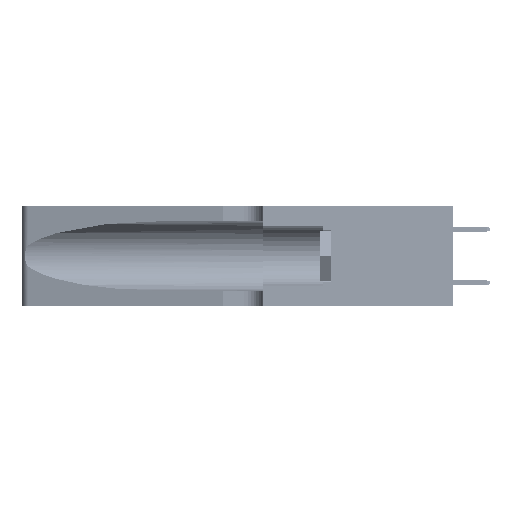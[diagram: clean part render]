
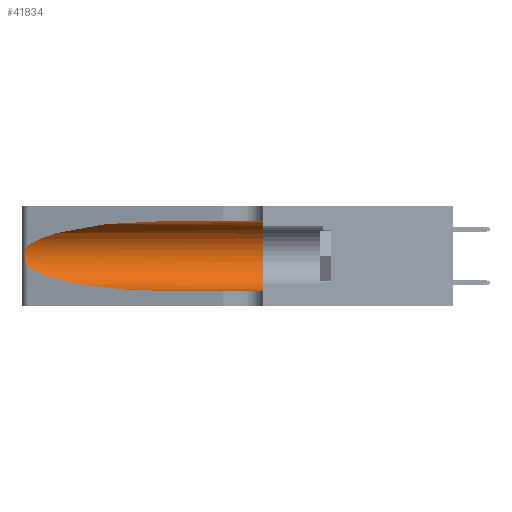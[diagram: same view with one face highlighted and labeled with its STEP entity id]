
A CAD part, left-side view. The second image highlights one B-rep face of the part: STEP entity #41834.
In plain terms, the highlighted cylindrical face has radius 3.308 mm (diameter 6.617 mm), a partial arc.
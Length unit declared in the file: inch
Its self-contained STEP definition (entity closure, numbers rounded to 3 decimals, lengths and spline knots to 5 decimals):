
#652 = FACE_OUTER_BOUND ( 'NONE', #35415, .T. ) ;
#1297 = ORIENTED_EDGE ( 'NONE', *, *, #24141, .F. ) ;
#1876 = EDGE_CURVE ( 'NONE', #30815, #19886, #15524, .T. ) ;
#3003 = CARTESIAN_POINT ( 'NONE',  ( 0.1305, 0.35, 0.31525 ) ) ;
#4019 = CARTESIAN_POINT ( 'NONE',  ( 0.1305, 0.72297, 0.31525 ) ) ;
#4290 = DIRECTION ( 'NONE',  ( 0., 0., -1. ) ) ;
#4959 = AXIS2_PLACEMENT_3D ( 'NONE', #5376, #8718, #4290 ) ;
#5376 = CARTESIAN_POINT ( 'NONE',  ( 0.1305, 1.61858, 0.185 ) ) ;
#7870 = CARTESIAN_POINT ( 'NONE',  ( 0.25854, 1.2359, 0.20912 ) ) ;
#8489 = VERTEX_POINT ( 'NONE', #17965 ) ;
#8718 = DIRECTION ( 'NONE',  ( 0., -1., 0. ) ) ;
#8997 = CYLINDRICAL_SURFACE ( 'NONE', #4959, 0.13025 ) ;
#9304 = CARTESIAN_POINT ( 'NONE',  ( 0.1305, 1.61858, 0.31525 ) ) ;
#9353 = B_SPLINE_CURVE_WITH_KNOTS ( 'NONE', 3,
 ( #24825, #20412, #28761, #49538, #7870, #41749, #29020, #24554, #20707, #45372, #40950, #37334, #45639, #45912 ),
 .UNSPECIFIED., .F., .F.,
 ( 4, 2, 2, 2, 2, 2, 4 ),
 ( 0., 0.00027, 0.00053, 0.00107, 0.0016, 0.00187, 0.00214 ),
 .UNSPECIFIED. ) ;
#12402 = DIRECTION ( 'NONE',  ( 0., 0., 1. ) ) ;
#15524 =( BOUNDED_CURVE ( )  B_SPLINE_CURVE ( 3, ( #38106, #30896, #17821, #39204 ),
 .UNSPECIFIED., .F., .F. ) 
 B_SPLINE_CURVE_WITH_KNOTS ( ( 4, 4 ),
 ( 3.44316, 4.71239 ),
 .UNSPECIFIED. ) 
 CURVE ( )  GEOMETRIC_REPRESENTATION_ITEM ( )  RATIONAL_B_SPLINE_CURVE ( ( 1., 0.87, 0.87, 1. ) ) 
 REPRESENTATION_ITEM ( '' )  );
#17821 = CARTESIAN_POINT ( 'NONE',  ( 0.18966, 0.96281, 0.05475 ) ) ;
#17965 = CARTESIAN_POINT ( 'NONE',  ( 0.1305, 0.35, 0.05475 ) ) ;
#19604 = CARTESIAN_POINT ( 'NONE',  ( 0.1305, 0.72297, 0.31525 ) ) ;
#19886 = VERTEX_POINT ( 'NONE', #39700 ) ;
#20171 = EDGE_CURVE ( 'NONE', #38620, #42905, #29901, .T. ) ;
#20412 = CARTESIAN_POINT ( 'NONE',  ( 0.25555, 1.22994, 0.2215 ) ) ;
#20615 = ORIENTED_EDGE ( 'NONE', *, *, #26371, .T. ) ;
#20707 = CARTESIAN_POINT ( 'NONE',  ( 0.26017, 1.23833, 0.17102 ) ) ;
#20763 = CARTESIAN_POINT ( 'NONE',  ( 0.25487, 1.22718, 0.22369 ) ) ;
#21088 = ORIENTED_EDGE ( 'NONE', *, *, #1876, .T. ) ;
#21697 = CARTESIAN_POINT ( 'NONE',  ( 0.1305, 1.61858, 0.05475 ) ) ;
#21811 = DIRECTION ( 'NONE',  ( 0., 1., 0. ) ) ;
#24032 = CARTESIAN_POINT ( 'NONE',  ( 0.25487, 1.22718, 0.22369 ) ) ;
#24141 = EDGE_CURVE ( 'NONE', #42905, #8489, #38104, .T. ) ;
#24554 = CARTESIAN_POINT ( 'NONE',  ( 0.26075, 1.23896, 0.178 ) ) ;
#24825 = CARTESIAN_POINT ( 'NONE',  ( 0.25487, 1.22718, 0.22369 ) ) ;
#26371 = EDGE_CURVE ( 'NONE', #19886, #8489, #42766, .T. ) ;
#28761 = CARTESIAN_POINT ( 'NONE',  ( 0.25639, 1.23184, 0.21858 ) ) ;
#29020 = CARTESIAN_POINT ( 'NONE',  ( 0.26075, 1.23896, 0.19203 ) ) ;
#29901 = LINE ( 'NONE', #9304, #48557 ) ;
#30815 = VERTEX_POINT ( 'NONE', #36262 ) ;
#30896 = CARTESIAN_POINT ( 'NONE',  ( 0.2373, 1.15595, 0.08982 ) ) ;
#31035 = AXIS2_PLACEMENT_3D ( 'NONE', #46506, #21811, #12402 ) ;
#32673 = CARTESIAN_POINT ( 'NONE',  ( 0.2373, 1.15595, 0.28018 ) ) ;
#33665 = ORIENTED_EDGE ( 'NONE', *, *, #45540, .T. ) ;
#35415 = EDGE_LOOP ( 'NONE', ( #37313, #33665, #21088, #20615, #1297, #46848 ) ) ;
#36262 = CARTESIAN_POINT ( 'NONE',  ( 0.25487, 1.22718, 0.14631 ) ) ;
#37313 = ORIENTED_EDGE ( 'NONE', *, *, #49734, .T. ) ;
#37334 = CARTESIAN_POINT ( 'NONE',  ( 0.25639, 1.23186, 0.15144 ) ) ;
#38104 = CIRCLE ( 'NONE', #31035, 0.13025 ) ;
#38106 = CARTESIAN_POINT ( 'NONE',  ( 0.25487, 1.22718, 0.14631 ) ) ;
#38620 = VERTEX_POINT ( 'NONE', #4019 ) ;
#39204 = CARTESIAN_POINT ( 'NONE',  ( 0.1305, 0.72297, 0.05475 ) ) ;
#39700 = CARTESIAN_POINT ( 'NONE',  ( 0.1305, 0.72297, 0.05475 ) ) ;
#40950 = CARTESIAN_POINT ( 'NONE',  ( 0.25789, 1.23486, 0.15765 ) ) ;
#41499 = CARTESIAN_POINT ( 'NONE',  ( 0.18966, 0.96281, 0.31525 ) ) ;
#41749 = CARTESIAN_POINT ( 'NONE',  ( 0.26018, 1.23835, 0.19895 ) ) ;
#41834 = ADVANCED_FACE ( 'NONE', ( #652 ), #8997, .F. ) ;
#42766 = LINE ( 'NONE', #21697, #47116 ) ;
#42905 = VERTEX_POINT ( 'NONE', #3003 ) ;
#45372 = CARTESIAN_POINT ( 'NONE',  ( 0.25856, 1.23593, 0.16098 ) ) ;
#45540 = EDGE_CURVE ( 'NONE', #53894, #30815, #9353, .T. ) ;
#45625 =( BOUNDED_CURVE ( )  B_SPLINE_CURVE ( 3, ( #19604, #41499, #32673, #24032 ),
 .UNSPECIFIED., .F., .F. ) 
 B_SPLINE_CURVE_WITH_KNOTS ( ( 4, 4 ),
 ( 1.5708, 2.84003 ),
 .UNSPECIFIED. ) 
 CURVE ( )  GEOMETRIC_REPRESENTATION_ITEM ( )  RATIONAL_B_SPLINE_CURVE ( ( 1., 0.87, 0.87, 1. ) ) 
 REPRESENTATION_ITEM ( '' )  );
#45639 = CARTESIAN_POINT ( 'NONE',  ( 0.25555, 1.22993, 0.14849 ) ) ;
#45912 = CARTESIAN_POINT ( 'NONE',  ( 0.25487, 1.22718, 0.14631 ) ) ;
#46506 = CARTESIAN_POINT ( 'NONE',  ( 0.1305, 0.35, 0.185 ) ) ;
#46848 = ORIENTED_EDGE ( 'NONE', *, *, #20171, .F. ) ;
#47116 = VECTOR ( 'NONE', #54715, 39.37008 ) ;
#48557 = VECTOR ( 'NONE', #50702, 39.37008 ) ;
#49538 = CARTESIAN_POINT ( 'NONE',  ( 0.25787, 1.23484, 0.2124 ) ) ;
#49734 = EDGE_CURVE ( 'NONE', #38620, #53894, #45625, .T. ) ;
#50702 = DIRECTION ( 'NONE',  ( 0., -1., 0. ) ) ;
#53894 = VERTEX_POINT ( 'NONE', #20763 ) ;
#54715 = DIRECTION ( 'NONE',  ( 0., -1., 0. ) ) ;
